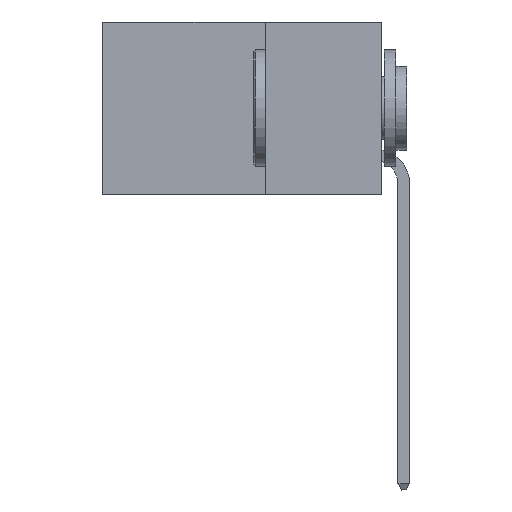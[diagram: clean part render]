
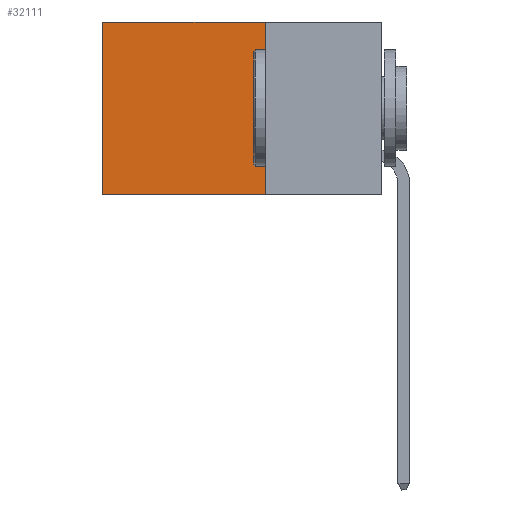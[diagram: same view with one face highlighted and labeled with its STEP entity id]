
A CAD part, left-side view. The second image highlights one B-rep face of the part: STEP entity #32111.
In plain terms, the highlighted planar face has unit normal (-1, 0, 0).
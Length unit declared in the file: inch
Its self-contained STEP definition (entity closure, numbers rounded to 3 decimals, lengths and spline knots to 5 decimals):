
#3216 = VECTOR ( 'NONE', #13173, 39.37008 ) ;
#6969 = ORIENTED_EDGE ( 'NONE', *, *, #9915, .F. ) ;
#7162 = LINE ( 'NONE', #19800, #41846 ) ;
#7165 = VERTEX_POINT ( 'NONE', #13918 ) ;
#9742 = VERTEX_POINT ( 'NONE', #40115 ) ;
#9915 = EDGE_CURVE ( 'NONE', #24603, #7165, #7162, .T. ) ;
#10523 = VECTOR ( 'NONE', #28676, 39.37008 ) ;
#11070 = VERTEX_POINT ( 'NONE', #11156 ) ;
#11156 = CARTESIAN_POINT ( 'NONE',  ( 0.2875, 0.6, 0. ) ) ;
#12837 = LINE ( 'NONE', #34684, #18578 ) ;
#13173 = DIRECTION ( 'NONE',  ( 0., 1., 0. ) ) ;
#13918 = CARTESIAN_POINT ( 'NONE',  ( 0.2875, 0.25, -0.37 ) ) ;
#14358 = CARTESIAN_POINT ( 'NONE',  ( 0.2875, 0.25, 0. ) ) ;
#16952 = DIRECTION ( 'NONE',  ( 0., 0., -1. ) ) ;
#17859 = DIRECTION ( 'NONE',  ( 0., 0., -1. ) ) ;
#18578 = VECTOR ( 'NONE', #20199, 39.37008 ) ;
#19800 = CARTESIAN_POINT ( 'NONE',  ( 0.2875, 0.25, 0. ) ) ;
#20199 = DIRECTION ( 'NONE',  ( 0., 0., -1. ) ) ;
#20971 = AXIS2_PLACEMENT_3D ( 'NONE', #27850, #21405, #17859 ) ;
#21405 = DIRECTION ( 'NONE',  ( 1., 0., 0. ) ) ;
#21753 = ORIENTED_EDGE ( 'NONE', *, *, #35846, .T. ) ;
#24603 = VERTEX_POINT ( 'NONE', #14358 ) ;
#25074 = EDGE_LOOP ( 'NONE', ( #40737, #27801, #6969, #21753 ) ) ;
#25276 = CARTESIAN_POINT ( 'NONE',  ( 0.2875, 0.25, 0. ) ) ;
#27783 = EDGE_CURVE ( 'NONE', #11070, #9742, #12837, .T. ) ;
#27801 = ORIENTED_EDGE ( 'NONE', *, *, #38049, .F. ) ;
#27850 = CARTESIAN_POINT ( 'NONE',  ( 0.2875, 0.25, 0. ) ) ;
#28676 = DIRECTION ( 'NONE',  ( 0., 1., 0. ) ) ;
#30505 = LINE ( 'NONE', #32846, #3216 ) ;
#32060 = LINE ( 'NONE', #25276, #10523 ) ;
#32111 = ADVANCED_FACE ( 'NONE', ( #33908 ), #38155, .F. ) ;
#32846 = CARTESIAN_POINT ( 'NONE',  ( 0.2875, 0.25, -0.37 ) ) ;
#33908 = FACE_OUTER_BOUND ( 'NONE', #25074, .T. ) ;
#34684 = CARTESIAN_POINT ( 'NONE',  ( 0.2875, 0.6, 0. ) ) ;
#35846 = EDGE_CURVE ( 'NONE', #24603, #11070, #32060, .T. ) ;
#38049 = EDGE_CURVE ( 'NONE', #7165, #9742, #30505, .T. ) ;
#38155 = PLANE ( 'NONE',  #20971 ) ;
#40115 = CARTESIAN_POINT ( 'NONE',  ( 0.2875, 0.6, -0.37 ) ) ;
#40737 = ORIENTED_EDGE ( 'NONE', *, *, #27783, .T. ) ;
#41846 = VECTOR ( 'NONE', #16952, 39.37008 ) ;
